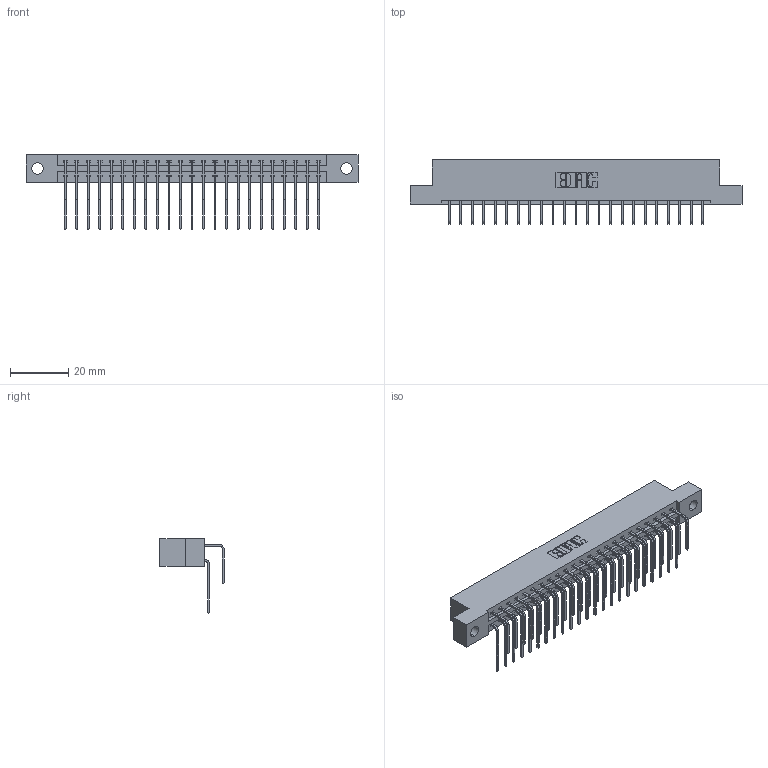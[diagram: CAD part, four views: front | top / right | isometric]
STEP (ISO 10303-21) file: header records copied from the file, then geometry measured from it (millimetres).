
FILE_DESCRIPTION (( 'STEP AP203' ), '1' );
FILE_NAME ('337-046-558-204.STEP', '2019-10-09T14:15:37', ( '' ), ( '' ), 'SwSTEP 2.0', 'SolidWorks 2016', '' );
FILE_SCHEMA (( 'CONFIG_CONTROL_DESIGN' ));
Length unit declared in the file: inch
Products named in the file (4): 337 Part_Flush Mounting Lugs - 0.156 Dia-TH; 337-046-558-204; 345-292-001_558 559 Tail - 1; 345-292-001_558 Tail - 2
Assembly tree (47 placements, depth 2):
  337-046-558-204
    337 Part_Flush Mounting Lugs - 0.156 Dia-TH
    345-292-001_558 559 Tail - 1  x23
    345-292-001_558 Tail - 2  x23
Bounding box: 114.15 x 22.17 x 25.53 mm (x, y, z)
Volume: 11954.4 mm3; surface area: 14459.7 mm2
Topology: 47 solids, 47 shells, 2690 faces, 7993 edges, 5266 vertices
Faces by surface type: plane 1910, cylinder 780
Entity records: 22077 total; most frequent: CARTESIAN_POINT 3781, ORIENTED_EDGE 3666, DIRECTION 3233, EDGE_CURVE 1833, LINE 1665, VECTOR 1665, VERTEX_POINT 1218, AXIS2_PLACEMENT_3D 784
